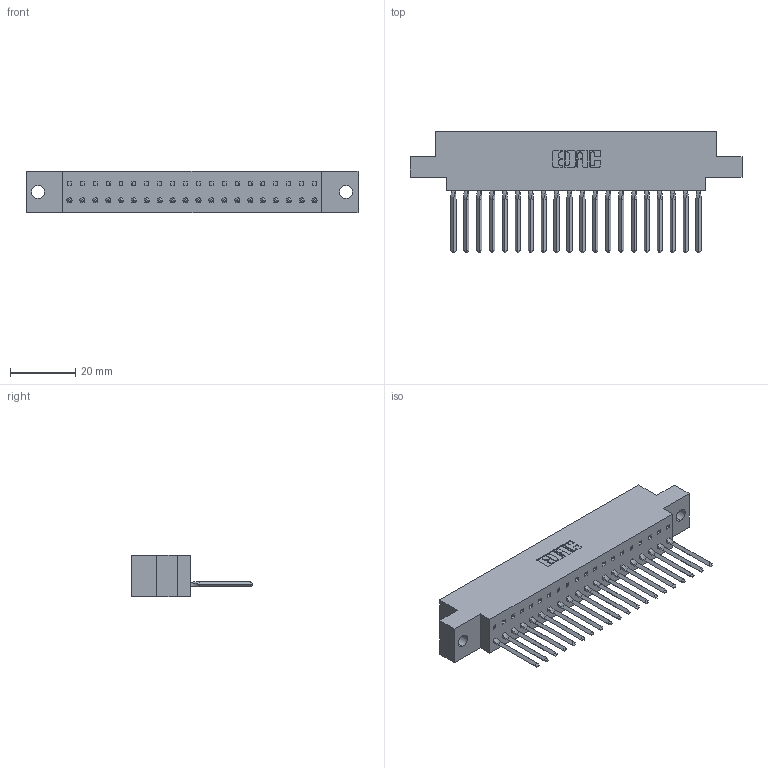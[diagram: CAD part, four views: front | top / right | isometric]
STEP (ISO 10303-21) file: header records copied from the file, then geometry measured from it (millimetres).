
FILE_DESCRIPTION (( 'STEP AP203' ), '1' );
FILE_NAME ('317-020-541-604.STEP', '2020-02-27T16:35:34', ( '' ), ( '' ), 'SwSTEP 2.0', 'SolidWorks 2016', '' );
FILE_SCHEMA (( 'CONFIG_CONTROL_DESIGN' ));
Length unit declared in the file: inch
Products named in the file (3): 317 Part_.156 Dia - TH; 317-020-541-604; 317-290-002_541
Assembly tree (21 placements, depth 2):
  317-020-541-604
    317 Part_.156 Dia - TH
    317-290-002_541  x20
Bounding box: 101.96 x 37.34 x 12.7 mm (x, y, z)
Volume: 15769.5 mm3; surface area: 21367.8 mm2
Topology: 21 solids, 21 shells, 3142 faces, 8955 edges, 5822 vertices
Faces by surface type: plane 2538, cylinder 524, bspline 80
Entity records: 32890 total; most frequent: CARTESIAN_POINT 6477, ORIENTED_EDGE 5750, DIRECTION 4707, EDGE_CURVE 2875, LINE 2511, VECTOR 2511, VERTEX_POINT 1908, AXIS2_PLACEMENT_3D 1098
